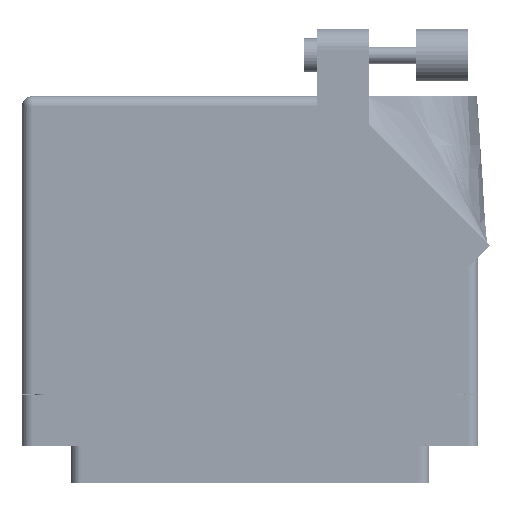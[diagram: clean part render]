
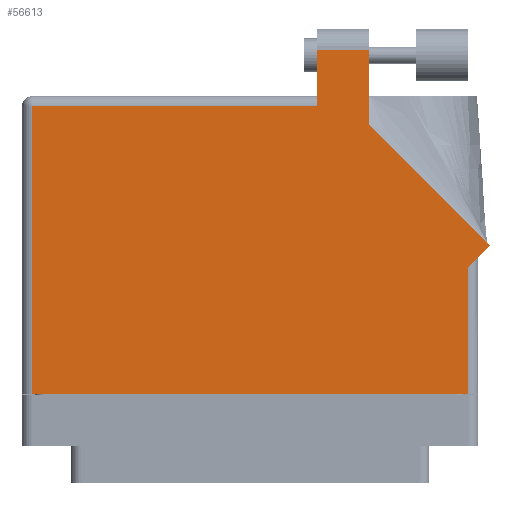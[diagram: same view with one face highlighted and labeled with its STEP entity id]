
A CAD part, front view. The second image highlights one B-rep face of the part: STEP entity #56613.
In plain terms, the highlighted face is planar.
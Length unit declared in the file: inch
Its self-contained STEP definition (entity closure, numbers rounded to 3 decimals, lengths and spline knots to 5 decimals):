
#1705 = ORIENTED_EDGE ( 'NONE', *, *, #48126, .T. ) ;
#1803 = ORIENTED_EDGE ( 'NONE', *, *, #66125, .T. ) ;
#2255 = CARTESIAN_POINT ( 'NONE',  ( 0.399, 1.613, 0.617 ) ) ;
#2323 = DIRECTION ( 'NONE',  ( -1., 0., 0. ) ) ;
#2802 = ORIENTED_EDGE ( 'NONE', *, *, #33112, .T. ) ;
#3063 = FACE_OUTER_BOUND ( 'NONE', #7019, .T. ) ;
#4219 = EDGE_CURVE ( 'NONE', #29141, #66782, #30130, .T. ) ;
#7019 = EDGE_LOOP ( 'NONE', ( #45094, #26024, #1803, #2802, #26958, #1705, #25053, #33950, #28508 ) ) ;
#9380 = CARTESIAN_POINT ( 'NONE',  ( 1.359, 0.715, 0.617 ) ) ;
#9937 = CARTESIAN_POINT ( 'NONE',  ( 1.42971, 0.78571, 0.617 ) ) ;
#10166 = DIRECTION ( 'NONE',  ( -0.707, 0.707, 0. ) ) ;
#10693 = LINE ( 'NONE', #43933, #43014 ) ;
#11561 = VERTEX_POINT ( 'NONE', #52629 ) ;
#11647 = DIRECTION ( 'NONE',  ( 0., 1., 0. ) ) ;
#12693 = LINE ( 'NONE', #9380, #18692 ) ;
#13186 = VERTEX_POINT ( 'NONE', #19179 ) ;
#13467 = DIRECTION ( 'NONE',  ( 0., 0., -1. ) ) ;
#14192 = PLANE ( 'NONE',  #70024 ) ;
#14820 = DIRECTION ( 'NONE',  ( 0.707, 0.707, 0. ) ) ;
#15700 = CARTESIAN_POINT ( 'NONE',  ( 1.297, -0.1, 0.617 ) ) ;
#16557 = LINE ( 'NONE', #38244, #50541 ) ;
#17420 = LINE ( 'NONE', #18247, #57332 ) ;
#17515 = VECTOR ( 'NONE', #10166, 39.37008 ) ;
#18247 = CARTESIAN_POINT ( 'NONE',  ( 0.399, 1.95, 0.617 ) ) ;
#18427 = CARTESIAN_POINT ( 'NONE',  ( 0.706, 1.50942, 0.617 ) ) ;
#18475 = CARTESIAN_POINT ( 'NONE',  ( 1.297, 0.653, 0.617 ) ) ;
#18692 = VECTOR ( 'NONE', #14820, 39.37008 ) ;
#19179 = CARTESIAN_POINT ( 'NONE',  ( 0.399, 1.95, 0.617 ) ) ;
#19547 = CARTESIAN_POINT ( 'NONE',  ( -1.297, -0.1, 0.617 ) ) ;
#20256 = DIRECTION ( 'NONE',  ( 0., -1., 0. ) ) ;
#20874 = VECTOR ( 'NONE', #38198, 39.37008 ) ;
#24390 = DIRECTION ( 'NONE',  ( -1., 0., 0. ) ) ;
#25053 = ORIENTED_EDGE ( 'NONE', *, *, #59460, .T. ) ;
#25743 = CARTESIAN_POINT ( 'NONE',  ( -1.297, -0.1, 0.617 ) ) ;
#26024 = ORIENTED_EDGE ( 'NONE', *, *, #38473, .T. ) ;
#26958 = ORIENTED_EDGE ( 'NONE', *, *, #60396, .T. ) ;
#28141 = VERTEX_POINT ( 'NONE', #29603 ) ;
#28508 = ORIENTED_EDGE ( 'NONE', *, *, #30531, .T. ) ;
#29141 = VERTEX_POINT ( 'NONE', #18427 ) ;
#29560 = DIRECTION ( 'NONE',  ( -1., 0., 0. ) ) ;
#29603 = CARTESIAN_POINT ( 'NONE',  ( 1.42971, 0.78571, 0.617 ) ) ;
#30130 = LINE ( 'NONE', #55086, #20874 ) ;
#30531 = EDGE_CURVE ( 'NONE', #28141, #29141, #54834, .T. ) ;
#31141 = VERTEX_POINT ( 'NONE', #2255 ) ;
#33112 = EDGE_CURVE ( 'NONE', #31141, #11561, #38529, .T. ) ;
#33296 = LINE ( 'NONE', #19547, #53809 ) ;
#33950 = ORIENTED_EDGE ( 'NONE', *, *, #54395, .T. ) ;
#34362 = CARTESIAN_POINT ( 'NONE',  ( -1.359, -0.1, 0.617 ) ) ;
#38076 = VERTEX_POINT ( 'NONE', #25743 ) ;
#38198 = DIRECTION ( 'NONE',  ( 0., 1., 0. ) ) ;
#38244 = CARTESIAN_POINT ( 'NONE',  ( 1.297, 0.715, 0.617 ) ) ;
#38473 = EDGE_CURVE ( 'NONE', #66782, #13186, #17420, .T. ) ;
#38529 = LINE ( 'NONE', #45292, #48804 ) ;
#40522 = CARTESIAN_POINT ( 'NONE',  ( -1.359, 1.675, 0.617 ) ) ;
#40713 = CARTESIAN_POINT ( 'NONE',  ( 0.706, 1.95, 0.617 ) ) ;
#43014 = VECTOR ( 'NONE', #49639, 39.37008 ) ;
#43933 = CARTESIAN_POINT ( 'NONE',  ( 0.399, 1.675, 0.617 ) ) ;
#45094 = ORIENTED_EDGE ( 'NONE', *, *, #4219, .T. ) ;
#45292 = CARTESIAN_POINT ( 'NONE',  ( -1.359, 1.613, 0.617 ) ) ;
#48126 = EDGE_CURVE ( 'NONE', #38076, #51811, #50002, .T. ) ;
#48804 = VECTOR ( 'NONE', #2323, 39.37008 ) ;
#49639 = DIRECTION ( 'NONE',  ( 0., -1., 0. ) ) ;
#50002 = LINE ( 'NONE', #34362, #59349 ) ;
#50541 = VECTOR ( 'NONE', #11647, 39.37008 ) ;
#51811 = VERTEX_POINT ( 'NONE', #15700 ) ;
#52629 = CARTESIAN_POINT ( 'NONE',  ( -1.297, 1.613, 0.617 ) ) ;
#53809 = VECTOR ( 'NONE', #20256, 39.37008 ) ;
#54395 = EDGE_CURVE ( 'NONE', #70311, #28141, #12693, .T. ) ;
#54834 = LINE ( 'NONE', #9937, #17515 ) ;
#55086 = CARTESIAN_POINT ( 'NONE',  ( 0.706, 1.50942, 0.617 ) ) ;
#56613 = ADVANCED_FACE ( 'NONE', ( #3063 ), #14192, .F. ) ;
#57332 = VECTOR ( 'NONE', #29560, 39.37008 ) ;
#59349 = VECTOR ( 'NONE', #67401, 39.37008 ) ;
#59460 = EDGE_CURVE ( 'NONE', #51811, #70311, #16557, .T. ) ;
#60396 = EDGE_CURVE ( 'NONE', #11561, #38076, #33296, .T. ) ;
#66125 = EDGE_CURVE ( 'NONE', #13186, #31141, #10693, .T. ) ;
#66782 = VERTEX_POINT ( 'NONE', #40713 ) ;
#67401 = DIRECTION ( 'NONE',  ( 1., 0., 0. ) ) ;
#70024 = AXIS2_PLACEMENT_3D ( 'NONE', #40522, #13467, #24390 ) ;
#70311 = VERTEX_POINT ( 'NONE', #18475 ) ;
